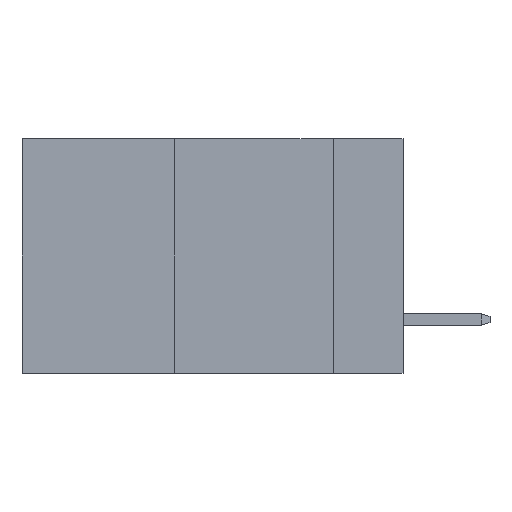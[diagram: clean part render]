
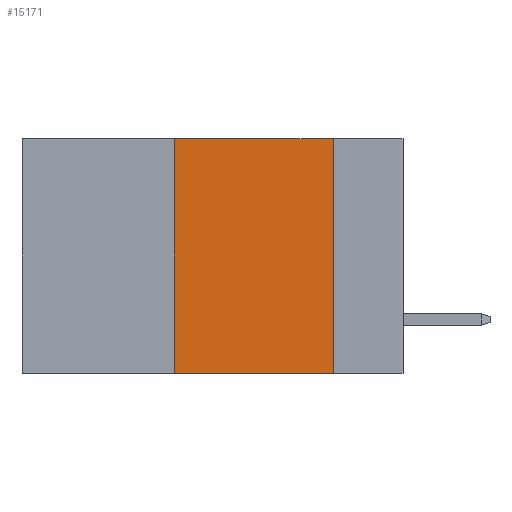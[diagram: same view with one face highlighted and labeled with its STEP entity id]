
A CAD part, left-side view. The second image highlights one B-rep face of the part: STEP entity #15171.
In plain terms, the highlighted planar face has unit normal (-1, 0, 0).
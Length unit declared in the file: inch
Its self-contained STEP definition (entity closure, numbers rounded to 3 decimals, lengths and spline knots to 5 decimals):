
#304 = CARTESIAN_POINT ( 'NONE',  ( 0., 0.11, 0. ) ) ;
#322 = EDGE_CURVE ( 'NONE', #7431, #11936, #1799, .T. ) ;
#1041 = CARTESIAN_POINT ( 'NONE',  ( 0., 0.11, -0.37 ) ) ;
#1096 = DIRECTION ( 'NONE',  ( 0., 0., -1. ) ) ;
#1799 = LINE ( 'NONE', #10220, #5896 ) ;
#2201 = DIRECTION ( 'NONE',  ( 0., -1., 0. ) ) ;
#2327 = ORIENTED_EDGE ( 'NONE', *, *, #3554, .T. ) ;
#2464 = DIRECTION ( 'NONE',  ( 0., 0., -1. ) ) ;
#3049 = DIRECTION ( 'NONE',  ( 0., 0., 1. ) ) ;
#3267 = EDGE_CURVE ( 'NONE', #3418, #9181, #5951, .T. ) ;
#3385 = ORIENTED_EDGE ( 'NONE', *, *, #5146, .F. ) ;
#3418 = VERTEX_POINT ( 'NONE', #304 ) ;
#3478 = DIRECTION ( 'NONE',  ( 1., 0., 0. ) ) ;
#3554 = EDGE_CURVE ( 'NONE', #7431, #9181, #14271, .T. ) ;
#4547 = AXIS2_PLACEMENT_3D ( 'NONE', #14364, #3478, #1096 ) ;
#4664 = PLANE ( 'NONE',  #4547 ) ;
#5146 = EDGE_CURVE ( 'NONE', #11936, #3418, #7992, .T. ) ;
#5680 = VECTOR ( 'NONE', #2201, 39.37008 ) ;
#5896 = VECTOR ( 'NONE', #3049, 39.37008 ) ;
#5934 = VECTOR ( 'NONE', #2464, 39.37008 ) ;
#5951 = LINE ( 'NONE', #13346, #5934 ) ;
#6517 = EDGE_LOOP ( 'NONE', ( #11620, #3385, #6589, #2327 ) ) ;
#6589 = ORIENTED_EDGE ( 'NONE', *, *, #322, .F. ) ;
#7431 = VERTEX_POINT ( 'NONE', #10527 ) ;
#7918 = DIRECTION ( 'NONE',  ( 0., -1., 0. ) ) ;
#7992 = LINE ( 'NONE', #13084, #5680 ) ;
#9181 = VERTEX_POINT ( 'NONE', #1041 ) ;
#9448 = FACE_OUTER_BOUND ( 'NONE', #6517, .T. ) ;
#10220 = CARTESIAN_POINT ( 'NONE',  ( 0., 0.36, 0. ) ) ;
#10527 = CARTESIAN_POINT ( 'NONE',  ( 0., 0.36, -0.37 ) ) ;
#11033 = VECTOR ( 'NONE', #7918, 39.37008 ) ;
#11620 = ORIENTED_EDGE ( 'NONE', *, *, #3267, .F. ) ;
#11936 = VERTEX_POINT ( 'NONE', #12916 ) ;
#12916 = CARTESIAN_POINT ( 'NONE',  ( 0., 0.36, 0. ) ) ;
#13084 = CARTESIAN_POINT ( 'NONE',  ( 0., 0.6, 0. ) ) ;
#13100 = CARTESIAN_POINT ( 'NONE',  ( 0., 0.6, -0.37 ) ) ;
#13346 = CARTESIAN_POINT ( 'NONE',  ( 0., 0.11, 0. ) ) ;
#14271 = LINE ( 'NONE', #13100, #11033 ) ;
#14364 = CARTESIAN_POINT ( 'NONE',  ( 0., 0.6, 0. ) ) ;
#15171 = ADVANCED_FACE ( 'NONE', ( #9448 ), #4664, .F. ) ;
